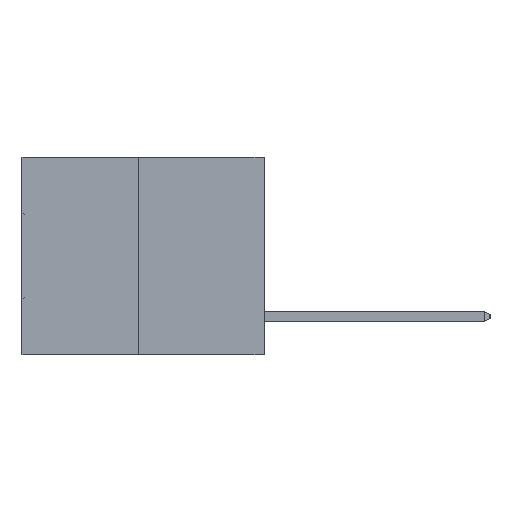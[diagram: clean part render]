
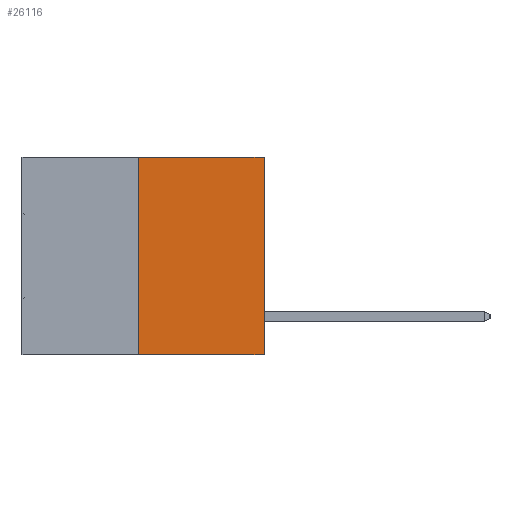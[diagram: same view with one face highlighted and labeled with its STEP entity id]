
A CAD part, left-side view. The second image highlights one B-rep face of the part: STEP entity #26116.
In plain terms, the highlighted planar face has unit normal (-1, 0, 0).
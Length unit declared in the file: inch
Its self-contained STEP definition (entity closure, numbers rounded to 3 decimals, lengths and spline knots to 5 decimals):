
#1498 = FACE_OUTER_BOUND ( 'NONE', #13932, .T. ) ;
#2648 = CARTESIAN_POINT ( 'NONE',  ( 0., 0., 0. ) ) ;
#2670 = CARTESIAN_POINT ( 'NONE',  ( 0., 0.312, 0. ) ) ;
#6569 = VERTEX_POINT ( 'NONE', #16012 ) ;
#6589 = VERTEX_POINT ( 'NONE', #21315 ) ;
#6664 = EDGE_CURVE ( 'NONE', #6569, #6589, #30950, .T. ) ;
#8388 = EDGE_CURVE ( 'NONE', #31292, #19855, #22628, .T. ) ;
#10311 = PLANE ( 'NONE',  #31971 ) ;
#11840 = DIRECTION ( 'NONE',  ( 0., 0., 1. ) ) ;
#12755 = CARTESIAN_POINT ( 'NONE',  ( 0., 0.6, 0. ) ) ;
#12944 = EDGE_CURVE ( 'NONE', #6589, #19855, #33425, .T. ) ;
#12979 = LINE ( 'NONE', #32745, #14695 ) ;
#13508 = ORIENTED_EDGE ( 'NONE', *, *, #16830, .F. ) ;
#13932 = EDGE_LOOP ( 'NONE', ( #13508, #25251, #26539, #23359 ) ) ;
#14695 = VECTOR ( 'NONE', #11840, 39.37008 ) ;
#15780 = DIRECTION ( 'NONE',  ( 0., 0., -1. ) ) ;
#16012 = CARTESIAN_POINT ( 'NONE',  ( 0., 0.312, -0.49 ) ) ;
#16470 = DIRECTION ( 'NONE',  ( 0., -1., 0. ) ) ;
#16830 = EDGE_CURVE ( 'NONE', #6569, #31292, #12979, .T. ) ;
#17030 = DIRECTION ( 'NONE',  ( 0., 0., 1. ) ) ;
#19855 = VERTEX_POINT ( 'NONE', #2648 ) ;
#21315 = CARTESIAN_POINT ( 'NONE',  ( 0., 0., -0.49 ) ) ;
#22628 = LINE ( 'NONE', #32344, #32912 ) ;
#23359 = ORIENTED_EDGE ( 'NONE', *, *, #8388, .F. ) ;
#23936 = VECTOR ( 'NONE', #16470, 39.37008 ) ;
#25251 = ORIENTED_EDGE ( 'NONE', *, *, #6664, .T. ) ;
#26116 = ADVANCED_FACE ( 'NONE', ( #1498 ), #10311, .F. ) ;
#26539 = ORIENTED_EDGE ( 'NONE', *, *, #12944, .T. ) ;
#26701 = CARTESIAN_POINT ( 'NONE',  ( 0., 0.6, -0.49 ) ) ;
#27726 = CARTESIAN_POINT ( 'NONE',  ( 0., 0., 0. ) ) ;
#28902 = DIRECTION ( 'NONE',  ( 1., 0., 0. ) ) ;
#30512 = VECTOR ( 'NONE', #17030, 39.37008 ) ;
#30950 = LINE ( 'NONE', #26701, #23936 ) ;
#31292 = VERTEX_POINT ( 'NONE', #2670 ) ;
#31971 = AXIS2_PLACEMENT_3D ( 'NONE', #12755, #28902, #15780 ) ;
#32344 = CARTESIAN_POINT ( 'NONE',  ( 0., 0.6, 0. ) ) ;
#32678 = DIRECTION ( 'NONE',  ( 0., -1., 0. ) ) ;
#32745 = CARTESIAN_POINT ( 'NONE',  ( 0., 0.312, -0.49 ) ) ;
#32912 = VECTOR ( 'NONE', #32678, 39.37008 ) ;
#33425 = LINE ( 'NONE', #27726, #30512 ) ;
